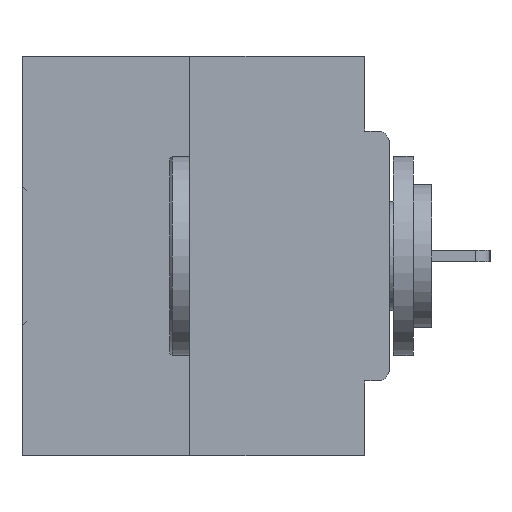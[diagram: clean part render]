
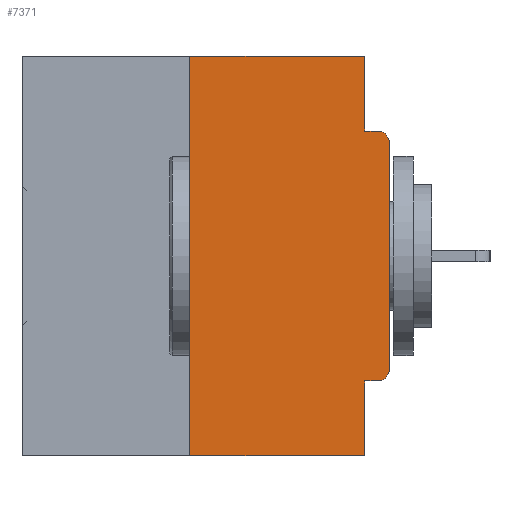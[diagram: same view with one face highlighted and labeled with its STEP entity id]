
A CAD part, left-side view. The second image highlights one B-rep face of the part: STEP entity #7371.
In plain terms, the highlighted planar face has unit normal (-1, 0, 0).
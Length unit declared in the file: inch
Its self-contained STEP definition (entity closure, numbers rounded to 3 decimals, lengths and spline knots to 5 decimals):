
#180 = DIRECTION ( 'NONE',  ( 0., 0., -1. ) ) ;
#257 = VECTOR ( 'NONE', #25186, 39.37008 ) ;
#774 = CARTESIAN_POINT ( 'NONE',  ( 0., 0.25, 0. ) ) ;
#863 = LINE ( 'NONE', #19397, #257 ) ;
#1123 = ORIENTED_EDGE ( 'NONE', *, *, #4362, .T. ) ;
#1599 = EDGE_CURVE ( 'NONE', #19558, #30843, #12889, .T. ) ;
#1980 = AXIS2_PLACEMENT_3D ( 'NONE', #26548, #38688, #29726 ) ;
#2430 = CARTESIAN_POINT ( 'NONE',  ( 0., 0., 0. ) ) ;
#3210 = DIRECTION ( 'NONE',  ( 0., 0., -1. ) ) ;
#3346 = CARTESIAN_POINT ( 'NONE',  ( 0., 0., -0.4065 ) ) ;
#3524 = VECTOR ( 'NONE', #22291, 39.37008 ) ;
#4296 = CARTESIAN_POINT ( 'NONE',  ( 0., 0.015, -0.4065 ) ) ;
#4362 = EDGE_CURVE ( 'NONE', #31185, #25529, #4496, .T. ) ;
#4401 = ORIENTED_EDGE ( 'NONE', *, *, #34970, .F. ) ;
#4496 = CIRCLE ( 'NONE', #1980, 0.015 ) ;
#5279 = ORIENTED_EDGE ( 'NONE', *, *, #35771, .F. ) ;
#5672 = CARTESIAN_POINT ( 'NONE',  ( 0., 0.46, -0.5 ) ) ;
#6532 = EDGE_CURVE ( 'NONE', #22226, #25529, #863, .T. ) ;
#6970 = FACE_OUTER_BOUND ( 'NONE', #10876, .T. ) ;
#7371 = ADVANCED_FACE ( 'NONE', ( #6970 ), #19105, .F. ) ;
#7529 = EDGE_CURVE ( 'NONE', #19558, #36509, #33311, .T. ) ;
#7635 = CARTESIAN_POINT ( 'NONE',  ( 0., 0.031, 0. ) ) ;
#7833 = LINE ( 'NONE', #28743, #11745 ) ;
#7884 = AXIS2_PLACEMENT_3D ( 'NONE', #31241, #18317, #180 ) ;
#8833 = CARTESIAN_POINT ( 'NONE',  ( 0., 0.46, 0. ) ) ;
#9016 = DIRECTION ( 'NONE',  ( 0., -1., 0. ) ) ;
#9175 = VECTOR ( 'NONE', #3210, 39.37008 ) ;
#10876 = EDGE_LOOP ( 'NONE', ( #21481, #5279, #34257, #38119, #19786, #33614, #19143, #1123, #35170, #4401 ) ) ;
#11745 = VECTOR ( 'NONE', #38087, 39.37008 ) ;
#12769 = CARTESIAN_POINT ( 'NONE',  ( 0., 0.031, -0.0935 ) ) ;
#12889 = LINE ( 'NONE', #3346, #38287 ) ;
#14607 = DIRECTION ( 'NONE',  ( 0., -1., 0. ) ) ;
#16858 = VERTEX_POINT ( 'NONE', #18244 ) ;
#17922 = VERTEX_POINT ( 'NONE', #20059 ) ;
#18244 = CARTESIAN_POINT ( 'NONE',  ( 0., 0.25, -0.5 ) ) ;
#18270 = VECTOR ( 'NONE', #26735, 39.37008 ) ;
#18317 = DIRECTION ( 'NONE',  ( 1., 0., 0. ) ) ;
#18588 = CARTESIAN_POINT ( 'NONE',  ( 0., 0.015, -0.0935 ) ) ;
#19105 = PLANE ( 'NONE',  #7884 ) ;
#19143 = ORIENTED_EDGE ( 'NONE', *, *, #31681, .T. ) ;
#19397 = CARTESIAN_POINT ( 'NONE',  ( 0., 0., -0.0935 ) ) ;
#19558 = VERTEX_POINT ( 'NONE', #4296 ) ;
#19709 = VERTEX_POINT ( 'NONE', #38293 ) ;
#19786 = ORIENTED_EDGE ( 'NONE', *, *, #1599, .F. ) ;
#20059 = CARTESIAN_POINT ( 'NONE',  ( 0., 0.031, -0.5 ) ) ;
#20233 = CARTESIAN_POINT ( 'NONE',  ( 0., 0.031, -0.4065 ) ) ;
#20675 = EDGE_CURVE ( 'NONE', #16858, #17922, #20992, .T. ) ;
#20992 = LINE ( 'NONE', #5672, #21758 ) ;
#21481 = ORIENTED_EDGE ( 'NONE', *, *, #31909, .F. ) ;
#21758 = VECTOR ( 'NONE', #14607, 39.37008 ) ;
#22226 = VERTEX_POINT ( 'NONE', #12769 ) ;
#22291 = DIRECTION ( 'NONE',  ( 0., 0., 1. ) ) ;
#22592 = CARTESIAN_POINT ( 'NONE',  ( 0., 0., -0.1085 ) ) ;
#23637 = DIRECTION ( 'NONE',  ( 0., 0., -1. ) ) ;
#25186 = DIRECTION ( 'NONE',  ( 0., -1., 0. ) ) ;
#25529 = VERTEX_POINT ( 'NONE', #18588 ) ;
#26548 = CARTESIAN_POINT ( 'NONE',  ( 0., 0.015, -0.1085 ) ) ;
#26735 = DIRECTION ( 'NONE',  ( 0., 0., 1. ) ) ;
#26970 = AXIS2_PLACEMENT_3D ( 'NONE', #38963, #30401, #23637 ) ;
#27085 = EDGE_CURVE ( 'NONE', #30843, #17922, #30508, .T. ) ;
#28743 = CARTESIAN_POINT ( 'NONE',  ( 0., 0.031, 0. ) ) ;
#29726 = DIRECTION ( 'NONE',  ( 0., 0., -1. ) ) ;
#29913 = CARTESIAN_POINT ( 'NONE',  ( 0., 0.031, -0.5 ) ) ;
#30401 = DIRECTION ( 'NONE',  ( -1., 0., 0. ) ) ;
#30508 = LINE ( 'NONE', #29913, #9175 ) ;
#30843 = VERTEX_POINT ( 'NONE', #20233 ) ;
#31013 = VECTOR ( 'NONE', #9016, 39.37008 ) ;
#31185 = VERTEX_POINT ( 'NONE', #22592 ) ;
#31241 = CARTESIAN_POINT ( 'NONE',  ( 0., 0.46, 0. ) ) ;
#31293 = CARTESIAN_POINT ( 'NONE',  ( 0., 0., -0.3915 ) ) ;
#31681 = EDGE_CURVE ( 'NONE', #36509, #31185, #34574, .T. ) ;
#31909 = EDGE_CURVE ( 'NONE', #19709, #36671, #36680, .T. ) ;
#33311 = CIRCLE ( 'NONE', #26970, 0.015 ) ;
#33614 = ORIENTED_EDGE ( 'NONE', *, *, #7529, .T. ) ;
#34257 = ORIENTED_EDGE ( 'NONE', *, *, #20675, .T. ) ;
#34574 = LINE ( 'NONE', #2430, #18270 ) ;
#34970 = EDGE_CURVE ( 'NONE', #36671, #22226, #7833, .T. ) ;
#35170 = ORIENTED_EDGE ( 'NONE', *, *, #6532, .F. ) ;
#35771 = EDGE_CURVE ( 'NONE', #16858, #19709, #37428, .T. ) ;
#36509 = VERTEX_POINT ( 'NONE', #31293 ) ;
#36608 = DIRECTION ( 'NONE',  ( 0., 1., 0. ) ) ;
#36671 = VERTEX_POINT ( 'NONE', #7635 ) ;
#36680 = LINE ( 'NONE', #8833, #31013 ) ;
#37428 = LINE ( 'NONE', #774, #3524 ) ;
#38087 = DIRECTION ( 'NONE',  ( 0., 0., -1. ) ) ;
#38119 = ORIENTED_EDGE ( 'NONE', *, *, #27085, .F. ) ;
#38287 = VECTOR ( 'NONE', #36608, 39.37008 ) ;
#38293 = CARTESIAN_POINT ( 'NONE',  ( 0., 0.25, 0. ) ) ;
#38688 = DIRECTION ( 'NONE',  ( -1., 0., 0. ) ) ;
#38963 = CARTESIAN_POINT ( 'NONE',  ( 0., 0.015, -0.3915 ) ) ;
